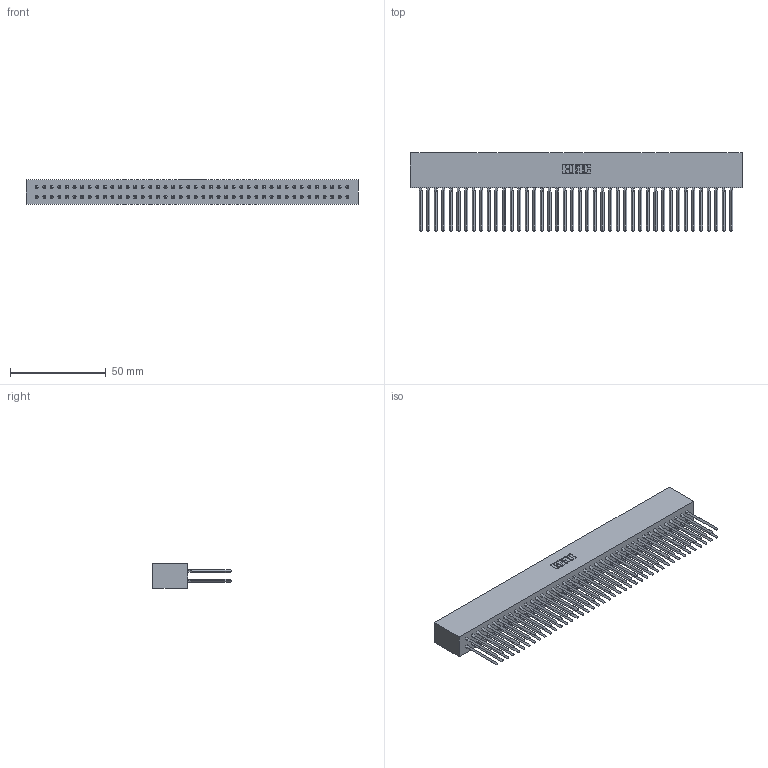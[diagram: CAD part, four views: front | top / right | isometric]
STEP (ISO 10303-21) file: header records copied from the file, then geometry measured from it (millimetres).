
FILE_DESCRIPTION (( 'STEP AP203' ), '1' );
FILE_NAME ('317-084-543-801.STEP', '2020-02-28T10:15:37', ( '' ), ( '' ), 'SwSTEP 2.0', 'SolidWorks 2016', '' );
FILE_SCHEMA (( 'CONFIG_CONTROL_DESIGN' ));
Products named in the file (3): 317 Part_Lugless; 317-290-001_543; 317-084-543-801
Assembly tree (85 placements, depth 2):
  317-084-543-801
    317 Part_Lugless
    317-290-001_543  x84
Bounding box: 173.63 x 41.15 x 12.7 mm (x, y, z)
Volume: 31352.9 mm3; surface area: 47841 mm2
Topology: 85 solids, 85 shells, 7566 faces, 20987 edges, 13514 vertices
Faces by surface type: plane 6182, cylinder 1048, bspline 336
Entity records: 60302 total; most frequent: CARTESIAN_POINT 10935, ORIENTED_EDGE 10434, DIRECTION 8695, EDGE_CURVE 5217, LINE 4969, VECTOR 4969, VERTEX_POINT 3471, AXIS2_PLACEMENT_3D 1863
